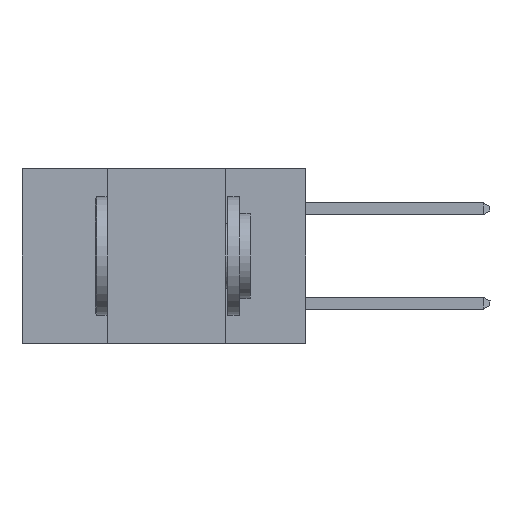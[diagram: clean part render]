
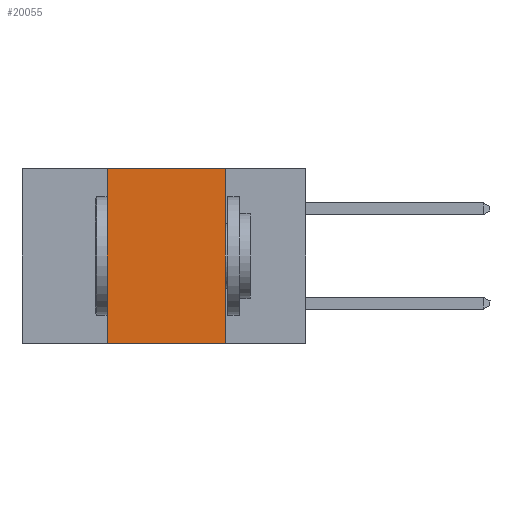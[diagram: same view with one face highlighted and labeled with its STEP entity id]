
A CAD part, left-side view. The second image highlights one B-rep face of the part: STEP entity #20055.
In plain terms, the highlighted planar face has unit normal (-1, 0, 0).
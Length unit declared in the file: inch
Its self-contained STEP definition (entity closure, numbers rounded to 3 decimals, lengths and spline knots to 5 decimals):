
#66 = DIRECTION ( 'NONE',  ( 1., 0., 0. ) ) ;
#1545 = CARTESIAN_POINT ( 'NONE',  ( 0., 0.42, 0. ) ) ;
#1552 = CARTESIAN_POINT ( 'NONE',  ( 0., 0.17, 0. ) ) ;
#1722 = EDGE_LOOP ( 'NONE', ( #20659, #13100, #10683, #12330 ) ) ;
#2687 = VECTOR ( 'NONE', #21124, 39.37008 ) ;
#3472 = DIRECTION ( 'NONE',  ( 0., 0., -1. ) ) ;
#3752 = VERTEX_POINT ( 'NONE', #10254 ) ;
#4226 = EDGE_CURVE ( 'NONE', #10706, #12311, #6377, .T. ) ;
#4256 = DIRECTION ( 'NONE',  ( 0., -1., 0. ) ) ;
#5966 = PLANE ( 'NONE',  #8423 ) ;
#6377 = LINE ( 'NONE', #13184, #21963 ) ;
#7823 = LINE ( 'NONE', #1552, #8402 ) ;
#8128 = DIRECTION ( 'NONE',  ( 0., -1., 0. ) ) ;
#8402 = VECTOR ( 'NONE', #3472, 39.37008 ) ;
#8423 = AXIS2_PLACEMENT_3D ( 'NONE', #15818, #66, #22940 ) ;
#9659 = EDGE_CURVE ( 'NONE', #10706, #3752, #22739, .T. ) ;
#9820 = CARTESIAN_POINT ( 'NONE',  ( 0., 0.17, 0. ) ) ;
#9894 = VECTOR ( 'NONE', #8128, 39.37008 ) ;
#10254 = CARTESIAN_POINT ( 'NONE',  ( 0., 0.42, 0. ) ) ;
#10683 = ORIENTED_EDGE ( 'NONE', *, *, #9659, .F. ) ;
#10706 = VERTEX_POINT ( 'NONE', #17171 ) ;
#10979 = FACE_OUTER_BOUND ( 'NONE', #1722, .T. ) ;
#12311 = VERTEX_POINT ( 'NONE', #19887 ) ;
#12330 = ORIENTED_EDGE ( 'NONE', *, *, #4226, .T. ) ;
#12403 = VERTEX_POINT ( 'NONE', #9820 ) ;
#13100 = ORIENTED_EDGE ( 'NONE', *, *, #20392, .F. ) ;
#13184 = CARTESIAN_POINT ( 'NONE',  ( 0., 0.6, -0.37 ) ) ;
#13795 = LINE ( 'NONE', #16996, #9894 ) ;
#15818 = CARTESIAN_POINT ( 'NONE',  ( 0., 0.6, 0. ) ) ;
#16996 = CARTESIAN_POINT ( 'NONE',  ( 0., 0.6, 0. ) ) ;
#17171 = CARTESIAN_POINT ( 'NONE',  ( 0., 0.42, -0.37 ) ) ;
#19887 = CARTESIAN_POINT ( 'NONE',  ( 0., 0.17, -0.37 ) ) ;
#20055 = ADVANCED_FACE ( 'NONE', ( #10979 ), #5966, .F. ) ;
#20392 = EDGE_CURVE ( 'NONE', #3752, #12403, #13795, .T. ) ;
#20659 = ORIENTED_EDGE ( 'NONE', *, *, #21928, .F. ) ;
#21124 = DIRECTION ( 'NONE',  ( 0., 0., 1. ) ) ;
#21928 = EDGE_CURVE ( 'NONE', #12403, #12311, #7823, .T. ) ;
#21963 = VECTOR ( 'NONE', #4256, 39.37008 ) ;
#22739 = LINE ( 'NONE', #1545, #2687 ) ;
#22940 = DIRECTION ( 'NONE',  ( 0., 0., -1. ) ) ;
